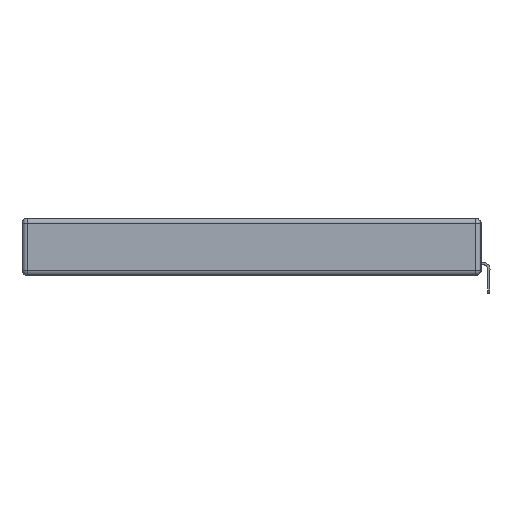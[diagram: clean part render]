
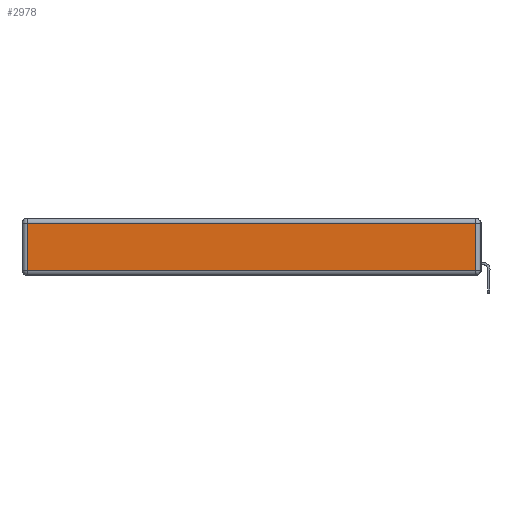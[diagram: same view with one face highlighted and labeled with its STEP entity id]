
A CAD part, left-side view. The second image highlights one B-rep face of the part: STEP entity #2978.
In plain terms, the highlighted planar face has unit normal (-1, 0, 0).
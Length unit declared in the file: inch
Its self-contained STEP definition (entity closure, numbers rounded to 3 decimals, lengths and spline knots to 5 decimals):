
#876 = ORIENTED_EDGE ( 'NONE', *, *, #21188, .T. ) ;
#1253 = VERTEX_POINT ( 'NONE', #4518 ) ;
#2025 = DIRECTION ( 'NONE',  ( -1., 0., 0. ) ) ;
#2273 = DIRECTION ( 'NONE',  ( 0., -1., 0. ) ) ;
#2978 = ADVANCED_FACE ( 'NONE', ( #5074 ), #15515, .T. ) ;
#3412 = EDGE_LOOP ( 'NONE', ( #8823, #17722, #876, #5279 ) ) ;
#3908 = CARTESIAN_POINT ( 'NONE',  ( 0., 0., -0.313 ) ) ;
#4129 = CARTESIAN_POINT ( 'NONE',  ( 0., 0.03, -0.03 ) ) ;
#4373 = CARTESIAN_POINT ( 'NONE',  ( 0., 0.03, -0.313 ) ) ;
#4420 = LINE ( 'NONE', #17662, #20343 ) ;
#4518 = CARTESIAN_POINT ( 'NONE',  ( 0., 2.72, -0.03 ) ) ;
#4845 = VECTOR ( 'NONE', #2273, 39.37008 ) ;
#5074 = FACE_OUTER_BOUND ( 'NONE', #3412, .T. ) ;
#5279 = ORIENTED_EDGE ( 'NONE', *, *, #18408, .T. ) ;
#5384 = CARTESIAN_POINT ( 'NONE',  ( 0., 0., -0.343 ) ) ;
#5758 = LINE ( 'NONE', #17227, #15815 ) ;
#6061 = DIRECTION ( 'NONE',  ( 0., 0., -1. ) ) ;
#8784 = DIRECTION ( 'NONE',  ( 0., 0., 1. ) ) ;
#8823 = ORIENTED_EDGE ( 'NONE', *, *, #10207, .T. ) ;
#9589 = VERTEX_POINT ( 'NONE', #18974 ) ;
#9697 = VERTEX_POINT ( 'NONE', #4373 ) ;
#10207 = EDGE_CURVE ( 'NONE', #9589, #9697, #18364, .T. ) ;
#10220 = VECTOR ( 'NONE', #19065, 39.37008 ) ;
#12464 = AXIS2_PLACEMENT_3D ( 'NONE', #5384, #2025, #8784 ) ;
#12504 = DIRECTION ( 'NONE',  ( 0., 0., 1. ) ) ;
#15252 = LINE ( 'NONE', #20856, #10220 ) ;
#15515 = PLANE ( 'NONE',  #12464 ) ;
#15815 = VECTOR ( 'NONE', #12504, 39.37008 ) ;
#17227 = CARTESIAN_POINT ( 'NONE',  ( 0., 0.03, -0.343 ) ) ;
#17662 = CARTESIAN_POINT ( 'NONE',  ( 0., 2.72, -0.343 ) ) ;
#17722 = ORIENTED_EDGE ( 'NONE', *, *, #19510, .T. ) ;
#18364 = LINE ( 'NONE', #3908, #4845 ) ;
#18408 = EDGE_CURVE ( 'NONE', #1253, #9589, #4420, .T. ) ;
#18974 = CARTESIAN_POINT ( 'NONE',  ( 0., 2.72, -0.313 ) ) ;
#19065 = DIRECTION ( 'NONE',  ( 0., 1., 0. ) ) ;
#19510 = EDGE_CURVE ( 'NONE', #9697, #20760, #5758, .T. ) ;
#20343 = VECTOR ( 'NONE', #6061, 39.37008 ) ;
#20760 = VERTEX_POINT ( 'NONE', #4129 ) ;
#20856 = CARTESIAN_POINT ( 'NONE',  ( 0., 2.75, -0.03 ) ) ;
#21188 = EDGE_CURVE ( 'NONE', #20760, #1253, #15252, .T. ) ;
